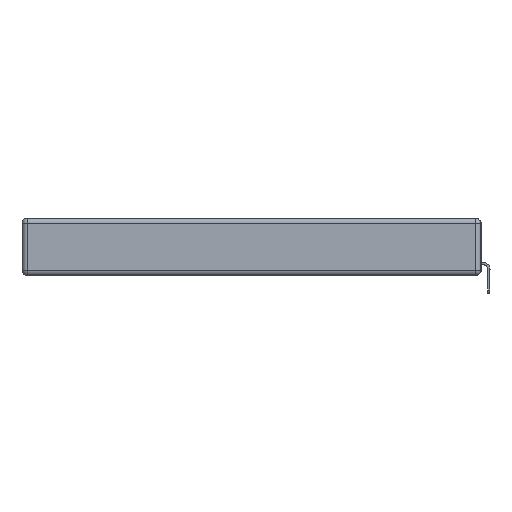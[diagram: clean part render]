
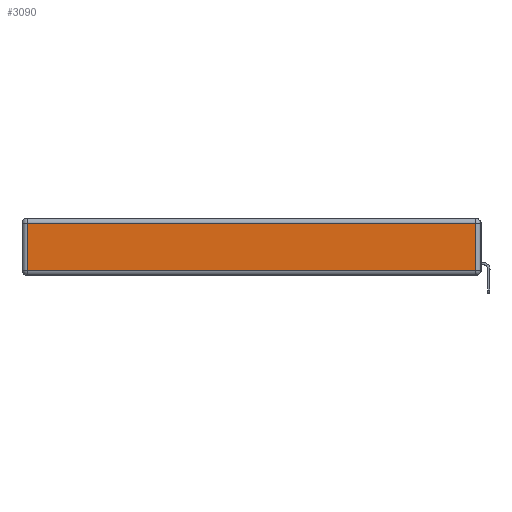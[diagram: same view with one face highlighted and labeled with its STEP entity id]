
A CAD part, left-side view. The second image highlights one B-rep face of the part: STEP entity #3090.
In plain terms, the highlighted planar face has unit normal (-1, 0, 0).
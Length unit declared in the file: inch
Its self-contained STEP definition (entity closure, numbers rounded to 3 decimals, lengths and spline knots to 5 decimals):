
#1072 = EDGE_CURVE ( 'NONE', #13887, #13645, #17599, .T. ) ;
#1214 = DIRECTION ( 'NONE',  ( 0., 1., 0. ) ) ;
#1459 = VECTOR ( 'NONE', #2884, 39.37008 ) ;
#1531 = AXIS2_PLACEMENT_3D ( 'NONE', #15873, #9108, #14521 ) ;
#2445 = LINE ( 'NONE', #14537, #15187 ) ;
#2770 = CARTESIAN_POINT ( 'NONE',  ( 0., 0.03, -0.343 ) ) ;
#2884 = DIRECTION ( 'NONE',  ( 0., 0., -1. ) ) ;
#3090 = ADVANCED_FACE ( 'NONE', ( #4936 ), #14631, .T. ) ;
#3264 = EDGE_CURVE ( 'NONE', #10527, #13887, #5704, .T. ) ;
#3334 = CARTESIAN_POINT ( 'NONE',  ( 0., 2.72, -0.313 ) ) ;
#4188 = DIRECTION ( 'NONE',  ( 0., 0., 1. ) ) ;
#4211 = CARTESIAN_POINT ( 'NONE',  ( 0., 2.72, -0.343 ) ) ;
#4936 = FACE_OUTER_BOUND ( 'NONE', #10501, .T. ) ;
#5326 = CARTESIAN_POINT ( 'NONE',  ( 0., 2.75, -0.03 ) ) ;
#5649 = VECTOR ( 'NONE', #4188, 39.37008 ) ;
#5704 = LINE ( 'NONE', #2770, #5649 ) ;
#6806 = CARTESIAN_POINT ( 'NONE',  ( 0., 0.03, -0.03 ) ) ;
#8485 = EDGE_CURVE ( 'NONE', #13645, #12755, #12411, .T. ) ;
#9108 = DIRECTION ( 'NONE',  ( -1., 0., 0. ) ) ;
#10458 = ORIENTED_EDGE ( 'NONE', *, *, #12023, .T. ) ;
#10501 = EDGE_LOOP ( 'NONE', ( #10458, #15299, #14451, #13046 ) ) ;
#10527 = VERTEX_POINT ( 'NONE', #15518 ) ;
#11795 = DIRECTION ( 'NONE',  ( 0., -1., 0. ) ) ;
#12023 = EDGE_CURVE ( 'NONE', #12755, #10527, #2445, .T. ) ;
#12411 = LINE ( 'NONE', #4211, #1459 ) ;
#12755 = VERTEX_POINT ( 'NONE', #3334 ) ;
#13046 = ORIENTED_EDGE ( 'NONE', *, *, #8485, .T. ) ;
#13380 = VECTOR ( 'NONE', #1214, 39.37008 ) ;
#13645 = VERTEX_POINT ( 'NONE', #14735 ) ;
#13887 = VERTEX_POINT ( 'NONE', #6806 ) ;
#14451 = ORIENTED_EDGE ( 'NONE', *, *, #1072, .T. ) ;
#14521 = DIRECTION ( 'NONE',  ( 0., 0., 1. ) ) ;
#14537 = CARTESIAN_POINT ( 'NONE',  ( 0., 0., -0.313 ) ) ;
#14631 = PLANE ( 'NONE',  #1531 ) ;
#14735 = CARTESIAN_POINT ( 'NONE',  ( 0., 2.72, -0.03 ) ) ;
#15187 = VECTOR ( 'NONE', #11795, 39.37008 ) ;
#15299 = ORIENTED_EDGE ( 'NONE', *, *, #3264, .T. ) ;
#15518 = CARTESIAN_POINT ( 'NONE',  ( 0., 0.03, -0.313 ) ) ;
#15873 = CARTESIAN_POINT ( 'NONE',  ( 0., 0., -0.343 ) ) ;
#17599 = LINE ( 'NONE', #5326, #13380 ) ;
